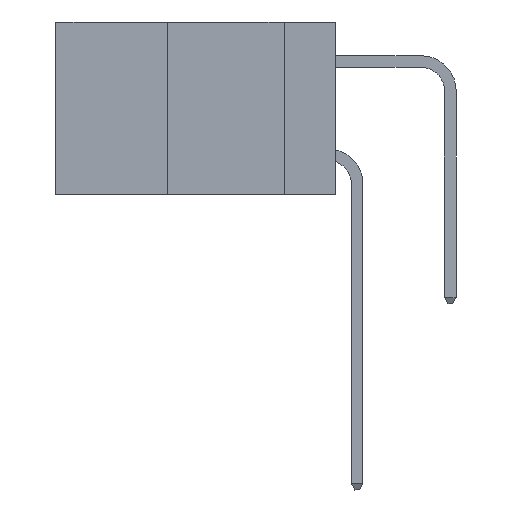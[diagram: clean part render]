
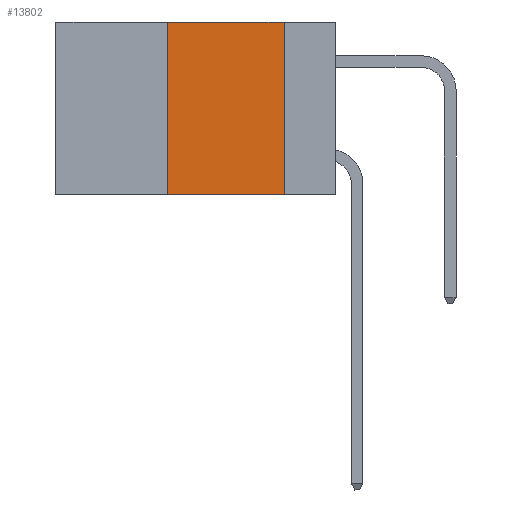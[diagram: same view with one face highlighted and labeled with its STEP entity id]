
A CAD part, left-side view. The second image highlights one B-rep face of the part: STEP entity #13802.
In plain terms, the highlighted planar face has unit normal (-1, 0, 0).
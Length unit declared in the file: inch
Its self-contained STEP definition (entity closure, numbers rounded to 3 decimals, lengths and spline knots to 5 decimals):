
#178 = PLANE ( 'NONE',  #5639 ) ;
#368 = VECTOR ( 'NONE', #6365, 39.37008 ) ;
#666 = CARTESIAN_POINT ( 'NONE',  ( 0., 0.36, -0.37 ) ) ;
#1083 = LINE ( 'NONE', #8191, #20440 ) ;
#1503 = VERTEX_POINT ( 'NONE', #1998 ) ;
#1998 = CARTESIAN_POINT ( 'NONE',  ( 0., 0.36, 0. ) ) ;
#2567 = EDGE_CURVE ( 'NONE', #18980, #1503, #1083, .T. ) ;
#2686 = CARTESIAN_POINT ( 'NONE',  ( 0., 0.11, -0.37 ) ) ;
#2821 = EDGE_CURVE ( 'NONE', #21105, #13192, #14986, .T. ) ;
#4084 = ORIENTED_EDGE ( 'NONE', *, *, #2567, .F. ) ;
#4678 = CARTESIAN_POINT ( 'NONE',  ( 0., 0.6, 0. ) ) ;
#4937 = DIRECTION ( 'NONE',  ( 0., 0., -1. ) ) ;
#5639 = AXIS2_PLACEMENT_3D ( 'NONE', #6638, #16765, #11602 ) ;
#6365 = DIRECTION ( 'NONE',  ( 0., -1., 0. ) ) ;
#6638 = CARTESIAN_POINT ( 'NONE',  ( 0., 0.6, 0. ) ) ;
#7426 = LINE ( 'NONE', #4678, #368 ) ;
#7528 = CARTESIAN_POINT ( 'NONE',  ( 0., 0.11, 0. ) ) ;
#8191 = CARTESIAN_POINT ( 'NONE',  ( 0., 0.36, 0. ) ) ;
#10088 = EDGE_CURVE ( 'NONE', #18980, #13192, #11344, .T. ) ;
#11344 = LINE ( 'NONE', #13661, #19704 ) ;
#11587 = VECTOR ( 'NONE', #4937, 39.37008 ) ;
#11602 = DIRECTION ( 'NONE',  ( 0., 0., -1. ) ) ;
#11795 = ORIENTED_EDGE ( 'NONE', *, *, #10088, .T. ) ;
#13192 = VERTEX_POINT ( 'NONE', #2686 ) ;
#13282 = CARTESIAN_POINT ( 'NONE',  ( 0., 0.11, 0. ) ) ;
#13661 = CARTESIAN_POINT ( 'NONE',  ( 0., 0.6, -0.37 ) ) ;
#13802 = ADVANCED_FACE ( 'NONE', ( #19799 ), #178, .F. ) ;
#14013 = DIRECTION ( 'NONE',  ( 0., -1., 0. ) ) ;
#14986 = LINE ( 'NONE', #13282, #11587 ) ;
#15974 = ORIENTED_EDGE ( 'NONE', *, *, #16319, .F. ) ;
#16319 = EDGE_CURVE ( 'NONE', #1503, #21105, #7426, .T. ) ;
#16765 = DIRECTION ( 'NONE',  ( 1., 0., 0. ) ) ;
#17833 = ORIENTED_EDGE ( 'NONE', *, *, #2821, .F. ) ;
#18035 = EDGE_LOOP ( 'NONE', ( #17833, #15974, #4084, #11795 ) ) ;
#18980 = VERTEX_POINT ( 'NONE', #666 ) ;
#19704 = VECTOR ( 'NONE', #14013, 39.37008 ) ;
#19799 = FACE_OUTER_BOUND ( 'NONE', #18035, .T. ) ;
#19900 = DIRECTION ( 'NONE',  ( 0., 0., 1. ) ) ;
#20440 = VECTOR ( 'NONE', #19900, 39.37008 ) ;
#21105 = VERTEX_POINT ( 'NONE', #7528 ) ;
